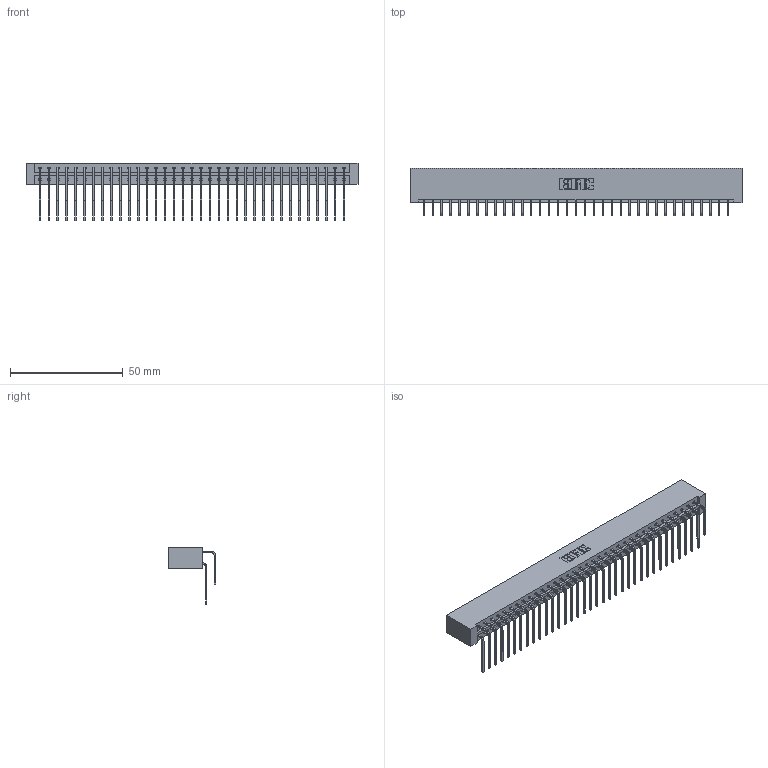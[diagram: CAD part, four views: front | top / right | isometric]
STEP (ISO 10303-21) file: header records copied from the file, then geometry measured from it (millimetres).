
FILE_DESCRIPTION (( 'STEP AP203' ), '1' );
FILE_NAME ('833-070-559-201.STEP', '2020-06-05T13:13:42', ( '' ), ( '' ), 'SwSTEP 2.0', 'SolidWorks 2020', '' );
FILE_SCHEMA (( 'CONFIG_CONTROL_DESIGN' ));
Length unit declared in the file: inch
Products named in the file (4): 345-292-001_558 559 Tail - 1; 345-292-001_559 Tail - 2; 833-070-559-201; 833 Part_Lugless
Assembly tree (71 placements, depth 2):
  833-070-559-201
    833 Part_Lugless
    345-292-001_558 559 Tail - 1  x35
    345-292-001_559 Tail - 2  x35
Bounding box: 146.94 x 20.9 x 25.53 mm (x, y, z)
Volume: 15972.2 mm3; surface area: 20843.7 mm2
Topology: 71 solids, 71 shells, 3886 faces, 11557 edges, 7610 vertices
Faces by surface type: plane 2726, cylinder 1160
Entity records: 24929 total; most frequent: CARTESIAN_POINT 4189, ORIENTED_EDGE 4074, DIRECTION 3565, EDGE_CURVE 2037, VECTOR 1877, LINE 1877, VERTEX_POINT 1354, AXIS2_PLACEMENT_3D 844
